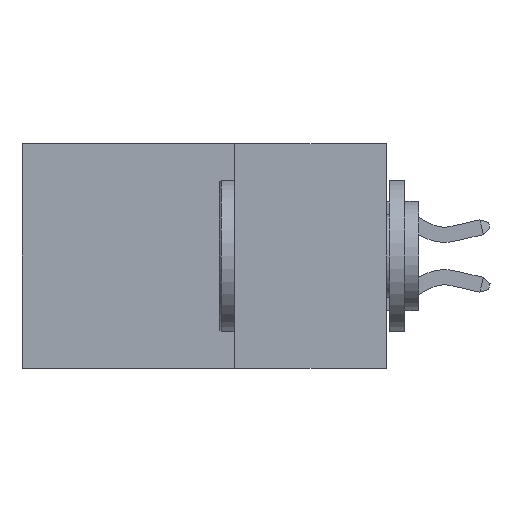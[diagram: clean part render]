
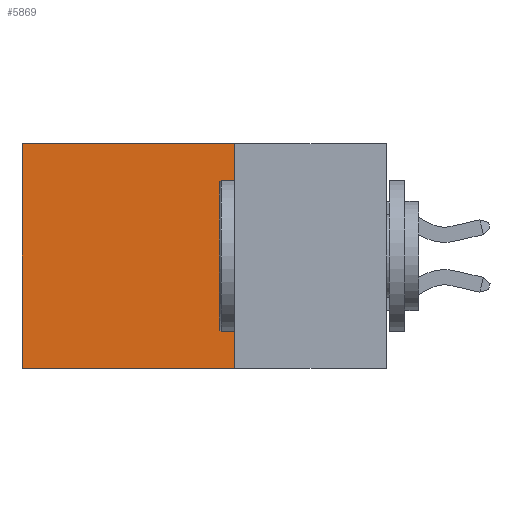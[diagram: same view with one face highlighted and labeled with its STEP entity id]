
A CAD part, left-side view. The second image highlights one B-rep face of the part: STEP entity #5869.
In plain terms, the highlighted planar face has unit normal (-1, 0, 0).
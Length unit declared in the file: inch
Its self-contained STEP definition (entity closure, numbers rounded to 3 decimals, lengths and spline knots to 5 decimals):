
#654 = DIRECTION ( 'NONE',  ( 0., 0., -1. ) ) ;
#1682 = LINE ( 'NONE', #12158, #7388 ) ;
#1691 = VECTOR ( 'NONE', #654, 39.37008 ) ;
#2276 = LINE ( 'NONE', #7933, #1691 ) ;
#3022 = LINE ( 'NONE', #18490, #15881 ) ;
#3556 = CARTESIAN_POINT ( 'NONE',  ( 0.298, 0.25, 0. ) ) ;
#4136 = VERTEX_POINT ( 'NONE', #5025 ) ;
#4574 = ORIENTED_EDGE ( 'NONE', *, *, #16678, .T. ) ;
#5025 = CARTESIAN_POINT ( 'NONE',  ( 0.298, 0.6, 0. ) ) ;
#5573 = ORIENTED_EDGE ( 'NONE', *, *, #23610, .F. ) ;
#5869 = ADVANCED_FACE ( 'NONE', ( #18808 ), #17202, .F. ) ;
#6261 = VERTEX_POINT ( 'NONE', #14687 ) ;
#7388 = VECTOR ( 'NONE', #21328, 39.37008 ) ;
#7933 = CARTESIAN_POINT ( 'NONE',  ( 0.298, 0.6, 0. ) ) ;
#7949 = ORIENTED_EDGE ( 'NONE', *, *, #20199, .F. ) ;
#8004 = VECTOR ( 'NONE', #16326, 39.37008 ) ;
#8086 = CARTESIAN_POINT ( 'NONE',  ( 0.298, 0.25, 0. ) ) ;
#8126 = CARTESIAN_POINT ( 'NONE',  ( 0.298, 0.25, -0.37 ) ) ;
#10122 = DIRECTION ( 'NONE',  ( 1., 0., 0. ) ) ;
#10504 = CARTESIAN_POINT ( 'NONE',  ( 0.298, 0.6, -0.37 ) ) ;
#12158 = CARTESIAN_POINT ( 'NONE',  ( 0.298, 0.25, -0.37 ) ) ;
#13240 = VERTEX_POINT ( 'NONE', #10504 ) ;
#13486 = LINE ( 'NONE', #3556, #8004 ) ;
#14687 = CARTESIAN_POINT ( 'NONE',  ( 0.298, 0.25, 0. ) ) ;
#15881 = VECTOR ( 'NONE', #22303, 39.37008 ) ;
#16326 = DIRECTION ( 'NONE',  ( 0., 1., 0. ) ) ;
#16339 = AXIS2_PLACEMENT_3D ( 'NONE', #8086, #10122, #19187 ) ;
#16678 = EDGE_CURVE ( 'NONE', #4136, #13240, #2276, .T. ) ;
#17202 = PLANE ( 'NONE',  #16339 ) ;
#17415 = ORIENTED_EDGE ( 'NONE', *, *, #22719, .T. ) ;
#17672 = EDGE_LOOP ( 'NONE', ( #4574, #5573, #7949, #17415 ) ) ;
#18490 = CARTESIAN_POINT ( 'NONE',  ( 0.298, 0.25, 0. ) ) ;
#18808 = FACE_OUTER_BOUND ( 'NONE', #17672, .T. ) ;
#19187 = DIRECTION ( 'NONE',  ( 0., 0., -1. ) ) ;
#20199 = EDGE_CURVE ( 'NONE', #6261, #21249, #3022, .T. ) ;
#21249 = VERTEX_POINT ( 'NONE', #8126 ) ;
#21328 = DIRECTION ( 'NONE',  ( 0., 1., 0. ) ) ;
#22303 = DIRECTION ( 'NONE',  ( 0., 0., -1. ) ) ;
#22719 = EDGE_CURVE ( 'NONE', #6261, #4136, #13486, .T. ) ;
#23610 = EDGE_CURVE ( 'NONE', #21249, #13240, #1682, .T. ) ;
